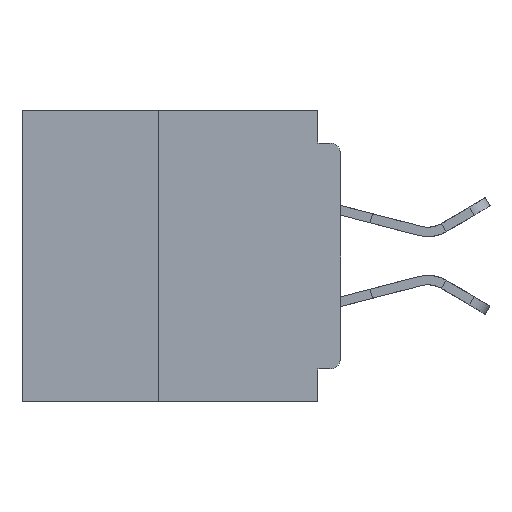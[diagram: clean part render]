
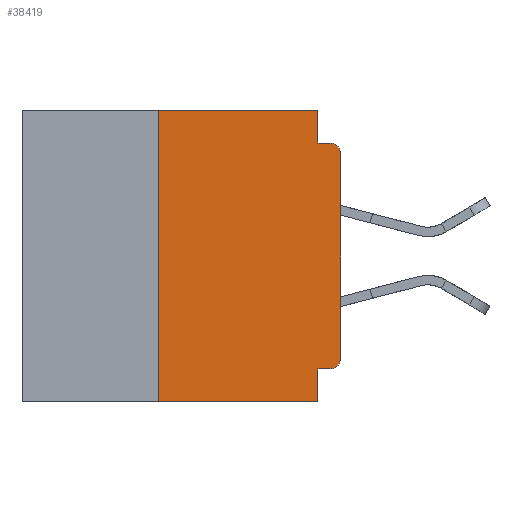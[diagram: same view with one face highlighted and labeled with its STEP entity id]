
A CAD part, left-side view. The second image highlights one B-rep face of the part: STEP entity #38419.
In plain terms, the highlighted planar face has unit normal (-1, 0, 0).
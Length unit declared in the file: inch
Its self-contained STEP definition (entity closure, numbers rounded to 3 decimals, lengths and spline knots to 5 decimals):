
#262 = CARTESIAN_POINT ( 'NONE',  ( 0., 0.031, -0.4 ) ) ;
#1025 = ORIENTED_EDGE ( 'NONE', *, *, #42258, .F. ) ;
#1356 = VERTEX_POINT ( 'NONE', #41801 ) ;
#2069 = VERTEX_POINT ( 'NONE', #20302 ) ;
#2346 = VECTOR ( 'NONE', #29201, 39.37008 ) ;
#2479 = EDGE_CURVE ( 'NONE', #46390, #2069, #30408, .T. ) ;
#2555 = VERTEX_POINT ( 'NONE', #11240 ) ;
#2766 = CARTESIAN_POINT ( 'NONE',  ( 0., 0., -0.34 ) ) ;
#3099 = LINE ( 'NONE', #15708, #21485 ) ;
#3505 = ORIENTED_EDGE ( 'NONE', *, *, #2479, .T. ) ;
#4553 = DIRECTION ( 'NONE',  ( 0., -1., 0. ) ) ;
#5086 = AXIS2_PLACEMENT_3D ( 'NONE', #42398, #46013, #24245 ) ;
#5210 = AXIS2_PLACEMENT_3D ( 'NONE', #19152, #44654, #22865 ) ;
#5602 = VECTOR ( 'NONE', #22507, 39.37008 ) ;
#6117 = CARTESIAN_POINT ( 'NONE',  ( 0., 0.015, -0.06 ) ) ;
#6299 = EDGE_CURVE ( 'NONE', #2555, #1356, #45413, .T. ) ;
#6904 = VERTEX_POINT ( 'NONE', #8197 ) ;
#7519 = ORIENTED_EDGE ( 'NONE', *, *, #40419, .F. ) ;
#7693 = VECTOR ( 'NONE', #4553, 39.37008 ) ;
#8197 = CARTESIAN_POINT ( 'NONE',  ( 0., 0., -0.06 ) ) ;
#8917 = FACE_OUTER_BOUND ( 'NONE', #41480, .T. ) ;
#9103 = ORIENTED_EDGE ( 'NONE', *, *, #9889, .T. ) ;
#9165 = VECTOR ( 'NONE', #10624, 39.37008 ) ;
#9819 = DIRECTION ( 'NONE',  ( 0., 0., -1. ) ) ;
#9889 = EDGE_CURVE ( 'NONE', #6904, #37918, #26354, .T. ) ;
#10624 = DIRECTION ( 'NONE',  ( 0., -1., 0. ) ) ;
#11240 = CARTESIAN_POINT ( 'NONE',  ( 0., 0.25, 0. ) ) ;
#12564 = EDGE_CURVE ( 'NONE', #22051, #6904, #3099, .T. ) ;
#14171 = CARTESIAN_POINT ( 'NONE',  ( 0., 0.015, -0.045 ) ) ;
#14579 = EDGE_CURVE ( 'NONE', #1356, #22664, #40127, .T. ) ;
#15708 = CARTESIAN_POINT ( 'NONE',  ( 0., 0., 0. ) ) ;
#16055 = DIRECTION ( 'NONE',  ( 0., 0., -1. ) ) ;
#16448 = DIRECTION ( 'NONE',  ( 0., -1., 0. ) ) ;
#16496 = CARTESIAN_POINT ( 'NONE',  ( 0., 0.437, -0.4 ) ) ;
#16523 = LINE ( 'NONE', #262, #5602 ) ;
#16842 = PLANE ( 'NONE',  #5086 ) ;
#18380 = CIRCLE ( 'NONE', #5210, 0.015 ) ;
#19152 = CARTESIAN_POINT ( 'NONE',  ( 0., 0.015, -0.34 ) ) ;
#19159 = VECTOR ( 'NONE', #23026, 39.37008 ) ;
#19276 = AXIS2_PLACEMENT_3D ( 'NONE', #6117, #31735, #9819 ) ;
#19320 = CARTESIAN_POINT ( 'NONE',  ( 0., 0., -0.355 ) ) ;
#19402 = DIRECTION ( 'NONE',  ( 0., 0., 1. ) ) ;
#20302 = CARTESIAN_POINT ( 'NONE',  ( 0., 0.031, -0.4 ) ) ;
#20787 = ORIENTED_EDGE ( 'NONE', *, *, #22262, .F. ) ;
#21485 = VECTOR ( 'NONE', #19402, 39.37008 ) ;
#21900 = LINE ( 'NONE', #25536, #2346 ) ;
#22051 = VERTEX_POINT ( 'NONE', #2766 ) ;
#22262 = EDGE_CURVE ( 'NONE', #38750, #2069, #16523, .T. ) ;
#22507 = DIRECTION ( 'NONE',  ( 0., 0., -1. ) ) ;
#22664 = VERTEX_POINT ( 'NONE', #43484 ) ;
#22865 = DIRECTION ( 'NONE',  ( 0., 0., -1. ) ) ;
#23026 = DIRECTION ( 'NONE',  ( 0., 1., 0. ) ) ;
#23209 = CARTESIAN_POINT ( 'NONE',  ( 0., 0.015, -0.355 ) ) ;
#24137 = VECTOR ( 'NONE', #16448, 39.37008 ) ;
#24245 = DIRECTION ( 'NONE',  ( 0., 0., -1. ) ) ;
#25029 = EDGE_CURVE ( 'NONE', #39478, #38750, #28883, .T. ) ;
#25536 = CARTESIAN_POINT ( 'NONE',  ( 0., 0.25, -0.4 ) ) ;
#26354 = CIRCLE ( 'NONE', #19276, 0.015 ) ;
#28799 = CARTESIAN_POINT ( 'NONE',  ( 0., 0.25, -0.4 ) ) ;
#28883 = LINE ( 'NONE', #19320, #19159 ) ;
#29201 = DIRECTION ( 'NONE',  ( 0., 0., 1. ) ) ;
#29274 = VECTOR ( 'NONE', #16055, 39.37008 ) ;
#30408 = LINE ( 'NONE', #16496, #24137 ) ;
#31735 = DIRECTION ( 'NONE',  ( -1., 0., 0. ) ) ;
#32133 = ORIENTED_EDGE ( 'NONE', *, *, #6299, .F. ) ;
#33293 = CARTESIAN_POINT ( 'NONE',  ( 0., 0.031, -0.355 ) ) ;
#33371 = EDGE_CURVE ( 'NONE', #39478, #22051, #18380, .T. ) ;
#33856 = CARTESIAN_POINT ( 'NONE',  ( 0., 0.437, 0. ) ) ;
#34103 = ORIENTED_EDGE ( 'NONE', *, *, #25029, .F. ) ;
#36248 = CARTESIAN_POINT ( 'NONE',  ( 0., 0., -0.045 ) ) ;
#37237 = LINE ( 'NONE', #36248, #9165 ) ;
#37918 = VERTEX_POINT ( 'NONE', #14171 ) ;
#37982 = CARTESIAN_POINT ( 'NONE',  ( 0., 0.031, 0. ) ) ;
#38419 = ADVANCED_FACE ( 'NONE', ( #8917 ), #16842, .F. ) ;
#38750 = VERTEX_POINT ( 'NONE', #33293 ) ;
#39284 = ORIENTED_EDGE ( 'NONE', *, *, #33371, .T. ) ;
#39478 = VERTEX_POINT ( 'NONE', #23209 ) ;
#40127 = LINE ( 'NONE', #37982, #29274 ) ;
#40419 = EDGE_CURVE ( 'NONE', #46390, #2555, #21900, .T. ) ;
#41480 = EDGE_LOOP ( 'NONE', ( #46758, #9103, #1025, #43409, #32133, #7519, #3505, #20787, #34103, #39284 ) ) ;
#41801 = CARTESIAN_POINT ( 'NONE',  ( 0., 0.031, 0. ) ) ;
#42258 = EDGE_CURVE ( 'NONE', #22664, #37918, #37237, .T. ) ;
#42398 = CARTESIAN_POINT ( 'NONE',  ( 0., 0.437, 0. ) ) ;
#43409 = ORIENTED_EDGE ( 'NONE', *, *, #14579, .F. ) ;
#43484 = CARTESIAN_POINT ( 'NONE',  ( 0., 0.031, -0.045 ) ) ;
#44654 = DIRECTION ( 'NONE',  ( -1., 0., 0. ) ) ;
#45413 = LINE ( 'NONE', #33856, #7693 ) ;
#46013 = DIRECTION ( 'NONE',  ( 1., 0., 0. ) ) ;
#46390 = VERTEX_POINT ( 'NONE', #28799 ) ;
#46758 = ORIENTED_EDGE ( 'NONE', *, *, #12564, .T. ) ;
